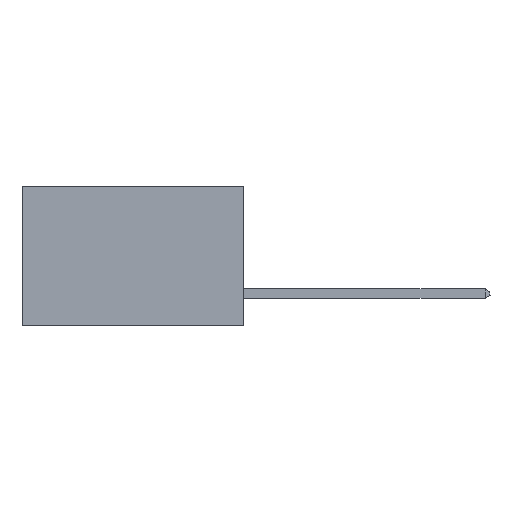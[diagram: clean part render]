
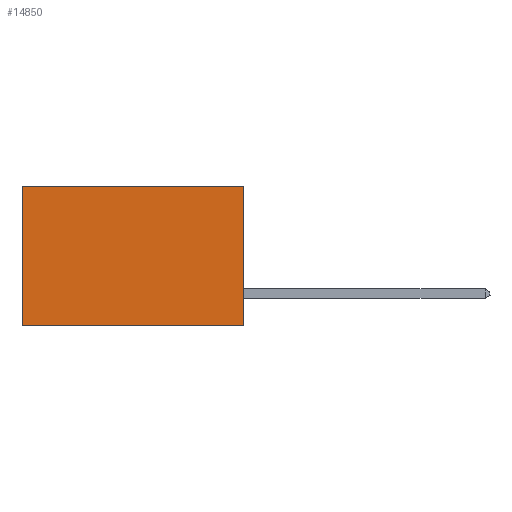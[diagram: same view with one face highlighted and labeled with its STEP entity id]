
A CAD part, left-side view. The second image highlights one B-rep face of the part: STEP entity #14850.
In plain terms, the highlighted planar face has unit normal (-1, 0, 0).
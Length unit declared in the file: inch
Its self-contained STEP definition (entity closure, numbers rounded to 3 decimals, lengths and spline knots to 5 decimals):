
#267 = CARTESIAN_POINT ( 'NONE',  ( 0.277, 0., 0. ) ) ;
#1407 = CARTESIAN_POINT ( 'NONE',  ( 0.277, 0.59, 0. ) ) ;
#1514 = DIRECTION ( 'NONE',  ( 0., 0., -1. ) ) ;
#1535 = EDGE_CURVE ( 'NONE', #3123, #11180, #4101, .T. ) ;
#2608 = VECTOR ( 'NONE', #4646, 39.37008 ) ;
#2778 = LINE ( 'NONE', #4963, #10593 ) ;
#3123 = VERTEX_POINT ( 'NONE', #267 ) ;
#3574 = EDGE_CURVE ( 'NONE', #3123, #5430, #2778, .T. ) ;
#3685 = ORIENTED_EDGE ( 'NONE', *, *, #6826, .F. ) ;
#3914 = ORIENTED_EDGE ( 'NONE', *, *, #1535, .F. ) ;
#4092 = VECTOR ( 'NONE', #11818, 39.37008 ) ;
#4101 = LINE ( 'NONE', #7359, #7737 ) ;
#4249 = VERTEX_POINT ( 'NONE', #16072 ) ;
#4646 = DIRECTION ( 'NONE',  ( 0., 1., 0. ) ) ;
#4963 = CARTESIAN_POINT ( 'NONE',  ( 0.277, 0., 0. ) ) ;
#5215 = DIRECTION ( 'NONE',  ( 0., 1., 0. ) ) ;
#5430 = VERTEX_POINT ( 'NONE', #1407 ) ;
#5777 = CARTESIAN_POINT ( 'NONE',  ( 0.277, 0., -0.37 ) ) ;
#6826 = EDGE_CURVE ( 'NONE', #11180, #4249, #15048, .T. ) ;
#7359 = CARTESIAN_POINT ( 'NONE',  ( 0.277, 0., -0.37 ) ) ;
#7737 = VECTOR ( 'NONE', #8362, 39.37008 ) ;
#8362 = DIRECTION ( 'NONE',  ( 0., 0., -1. ) ) ;
#10247 = CARTESIAN_POINT ( 'NONE',  ( 0.277, 0.59, -0.37 ) ) ;
#10593 = VECTOR ( 'NONE', #5215, 39.37008 ) ;
#10918 = DIRECTION ( 'NONE',  ( 1., 0., 0. ) ) ;
#11180 = VERTEX_POINT ( 'NONE', #17487 ) ;
#11818 = DIRECTION ( 'NONE',  ( 0., 0., -1. ) ) ;
#12422 = LINE ( 'NONE', #10247, #4092 ) ;
#13957 = CARTESIAN_POINT ( 'NONE',  ( 0.277, 0., -0.37 ) ) ;
#14850 = ADVANCED_FACE ( 'NONE', ( #19865 ), #18558, .F. ) ;
#14873 = AXIS2_PLACEMENT_3D ( 'NONE', #13957, #10918, #1514 ) ;
#15048 = LINE ( 'NONE', #5777, #2608 ) ;
#15874 = EDGE_LOOP ( 'NONE', ( #19627, #3685, #3914, #16064 ) ) ;
#16064 = ORIENTED_EDGE ( 'NONE', *, *, #3574, .T. ) ;
#16072 = CARTESIAN_POINT ( 'NONE',  ( 0.277, 0.59, -0.37 ) ) ;
#17487 = CARTESIAN_POINT ( 'NONE',  ( 0.277, 0., -0.37 ) ) ;
#18558 = PLANE ( 'NONE',  #14873 ) ;
#19585 = EDGE_CURVE ( 'NONE', #5430, #4249, #12422, .T. ) ;
#19627 = ORIENTED_EDGE ( 'NONE', *, *, #19585, .T. ) ;
#19865 = FACE_OUTER_BOUND ( 'NONE', #15874, .T. ) ;
